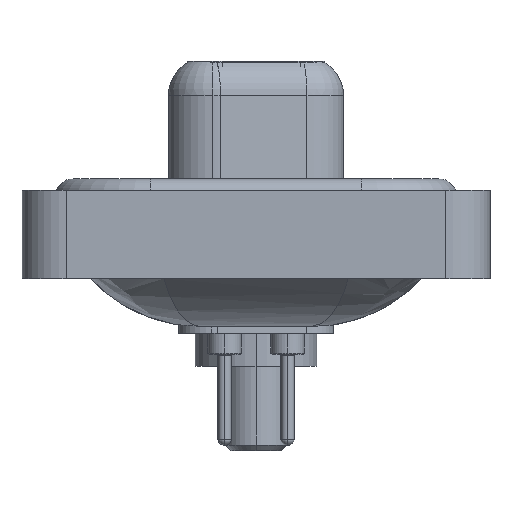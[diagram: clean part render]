
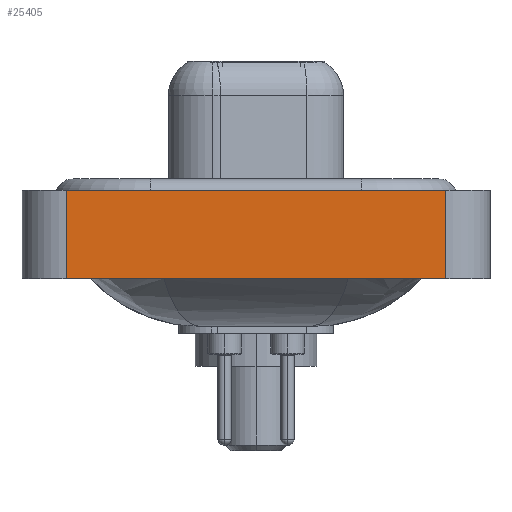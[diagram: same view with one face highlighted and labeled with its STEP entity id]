
A CAD part, left-side view. The second image highlights one B-rep face of the part: STEP entity #25405.
In plain terms, the highlighted planar face has unit normal (-1, 0, 0).
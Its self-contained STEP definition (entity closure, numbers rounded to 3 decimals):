
#336 = EDGE_CURVE ( 'NONE', #11140, #1869, #665, .T. ) ;
#665 = LINE ( 'NONE', #4789, #25010 ) ;
#1682 = DIRECTION ( 'NONE',  ( 0., -1., 0. ) ) ;
#1757 = CARTESIAN_POINT ( 'NONE',  ( -7.35, 8.55, -3.6 ) ) ;
#1869 = VERTEX_POINT ( 'NONE', #2426 ) ;
#2426 = CARTESIAN_POINT ( 'NONE',  ( -7.35, 8.55, 0.4 ) ) ;
#3563 = LINE ( 'NONE', #17843, #23882 ) ;
#3758 = LINE ( 'NONE', #16050, #13053 ) ;
#4110 = FACE_OUTER_BOUND ( 'NONE', #14336, .T. ) ;
#4789 = CARTESIAN_POINT ( 'NONE',  ( -7.35, 8.55, -3.6 ) ) ;
#5624 = DIRECTION ( 'NONE',  ( 0., 0., 1. ) ) ;
#6690 = VERTEX_POINT ( 'NONE', #10296 ) ;
#6820 = ORIENTED_EDGE ( 'NONE', *, *, #8354, .T. ) ;
#7829 = PLANE ( 'NONE',  #25214 ) ;
#8354 = EDGE_CURVE ( 'NONE', #11140, #11744, #21904, .T. ) ;
#8906 = ORIENTED_EDGE ( 'NONE', *, *, #12522, .T. ) ;
#9287 = DIRECTION ( 'NONE',  ( 0., 0., 1. ) ) ;
#10296 = CARTESIAN_POINT ( 'NONE',  ( -7.35, -8.55, 0.4 ) ) ;
#11140 = VERTEX_POINT ( 'NONE', #1757 ) ;
#11498 = ORIENTED_EDGE ( 'NONE', *, *, #336, .F. ) ;
#11744 = VERTEX_POINT ( 'NONE', #20672 ) ;
#12125 = DIRECTION ( 'NONE',  ( -1., 0., 0. ) ) ;
#12522 = EDGE_CURVE ( 'NONE', #11744, #6690, #3758, .T. ) ;
#13053 = VECTOR ( 'NONE', #5624, 1000. ) ;
#14044 = DIRECTION ( 'NONE',  ( 0., -1., 0. ) ) ;
#14336 = EDGE_LOOP ( 'NONE', ( #8906, #26198, #11498, #6820 ) ) ;
#16050 = CARTESIAN_POINT ( 'NONE',  ( -7.35, -8.55, -3.6 ) ) ;
#17843 = CARTESIAN_POINT ( 'NONE',  ( -7.35, -8.55, 0.4 ) ) ;
#20672 = CARTESIAN_POINT ( 'NONE',  ( -7.35, -8.55, -3.6 ) ) ;
#21751 = EDGE_CURVE ( 'NONE', #1869, #6690, #3563, .T. ) ;
#21904 = LINE ( 'NONE', #24301, #24306 ) ;
#22264 = DIRECTION ( 'NONE',  ( 0., 0., 1. ) ) ;
#23882 = VECTOR ( 'NONE', #1682, 1000. ) ;
#24301 = CARTESIAN_POINT ( 'NONE',  ( -7.35, -8.55, -3.6 ) ) ;
#24306 = VECTOR ( 'NONE', #14044, 1000. ) ;
#25010 = VECTOR ( 'NONE', #9287, 1000. ) ;
#25214 = AXIS2_PLACEMENT_3D ( 'NONE', #26269, #12125, #22264 ) ;
#25405 = ADVANCED_FACE ( 'NONE', ( #4110 ), #7829, .T. ) ;
#26198 = ORIENTED_EDGE ( 'NONE', *, *, #21751, .F. ) ;
#26269 = CARTESIAN_POINT ( 'NONE',  ( -7.35, -8.55, -3.6 ) ) ;
